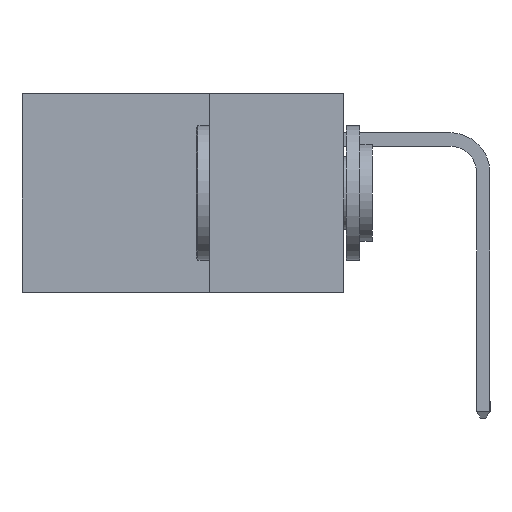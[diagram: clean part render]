
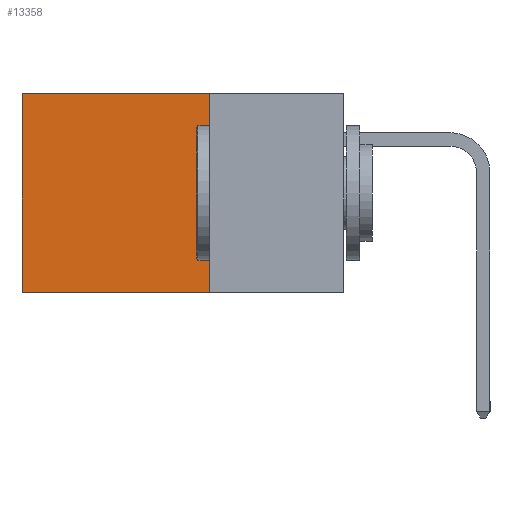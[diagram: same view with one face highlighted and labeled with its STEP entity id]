
A CAD part, left-side view. The second image highlights one B-rep face of the part: STEP entity #13358.
In plain terms, the highlighted planar face has unit normal (-1, 0, 0).
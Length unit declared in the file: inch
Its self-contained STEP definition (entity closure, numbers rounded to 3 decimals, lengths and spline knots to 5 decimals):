
#3512 = VECTOR ( 'NONE', #13110, 39.37008 ) ;
#3947 = FACE_OUTER_BOUND ( 'NONE', #7834, .T. ) ;
#5637 = LINE ( 'NONE', #6879, #15143 ) ;
#5931 = DIRECTION ( 'NONE',  ( 0., 0., -1. ) ) ;
#6292 = VERTEX_POINT ( 'NONE', #11056 ) ;
#6453 = VECTOR ( 'NONE', #22317, 39.37008 ) ;
#6879 = CARTESIAN_POINT ( 'NONE',  ( 0.2615, 0.25, 0. ) ) ;
#6955 = DIRECTION ( 'NONE',  ( 0., 1., 0. ) ) ;
#7834 = EDGE_LOOP ( 'NONE', ( #12014, #16307, #21974, #19248 ) ) ;
#8797 = VECTOR ( 'NONE', #10375, 39.37008 ) ;
#9190 = EDGE_CURVE ( 'NONE', #6292, #21381, #5637, .T. ) ;
#10375 = DIRECTION ( 'NONE',  ( 0., 0., -1. ) ) ;
#10915 = CARTESIAN_POINT ( 'NONE',  ( 0.2615, 0.6, -0.37 ) ) ;
#11056 = CARTESIAN_POINT ( 'NONE',  ( 0.2615, 0.25, 0. ) ) ;
#11281 = CARTESIAN_POINT ( 'NONE',  ( 0.2615, 0.25, -0.37 ) ) ;
#11492 = LINE ( 'NONE', #14782, #6453 ) ;
#12014 = ORIENTED_EDGE ( 'NONE', *, *, #21747, .T. ) ;
#13110 = DIRECTION ( 'NONE',  ( 0., 1., 0. ) ) ;
#13358 = ADVANCED_FACE ( 'NONE', ( #3947 ), #15400, .F. ) ;
#13494 = CARTESIAN_POINT ( 'NONE',  ( 0.2615, 0.25, -0.37 ) ) ;
#13867 = LINE ( 'NONE', #17800, #8797 ) ;
#14613 = EDGE_CURVE ( 'NONE', #23092, #20893, #18023, .T. ) ;
#14782 = CARTESIAN_POINT ( 'NONE',  ( 0.2615, 0.25, -0.37 ) ) ;
#15143 = VECTOR ( 'NONE', #6955, 39.37008 ) ;
#15400 = PLANE ( 'NONE',  #18833 ) ;
#15952 = EDGE_CURVE ( 'NONE', #6292, #23092, #11492, .T. ) ;
#16307 = ORIENTED_EDGE ( 'NONE', *, *, #14613, .F. ) ;
#17263 = DIRECTION ( 'NONE',  ( 1., 0., 0. ) ) ;
#17800 = CARTESIAN_POINT ( 'NONE',  ( 0.2615, 0.6, -0.37 ) ) ;
#18023 = LINE ( 'NONE', #11281, #3512 ) ;
#18833 = AXIS2_PLACEMENT_3D ( 'NONE', #13494, #17263, #5931 ) ;
#19248 = ORIENTED_EDGE ( 'NONE', *, *, #9190, .T. ) ;
#19890 = CARTESIAN_POINT ( 'NONE',  ( 0.2615, 0.6, 0. ) ) ;
#20893 = VERTEX_POINT ( 'NONE', #10915 ) ;
#21381 = VERTEX_POINT ( 'NONE', #19890 ) ;
#21747 = EDGE_CURVE ( 'NONE', #21381, #20893, #13867, .T. ) ;
#21974 = ORIENTED_EDGE ( 'NONE', *, *, #15952, .F. ) ;
#22317 = DIRECTION ( 'NONE',  ( 0., 0., -1. ) ) ;
#23092 = VERTEX_POINT ( 'NONE', #23949 ) ;
#23949 = CARTESIAN_POINT ( 'NONE',  ( 0.2615, 0.25, -0.37 ) ) ;
